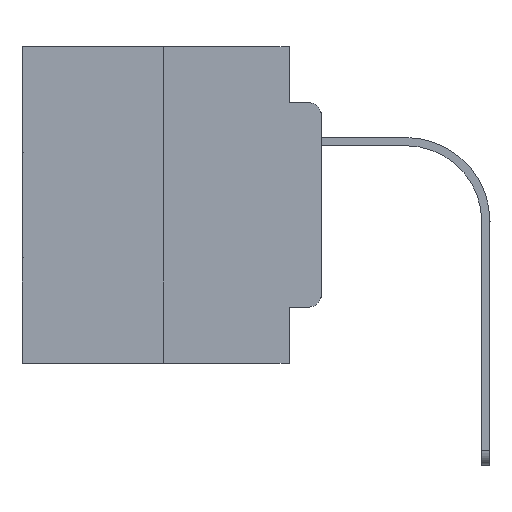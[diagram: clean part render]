
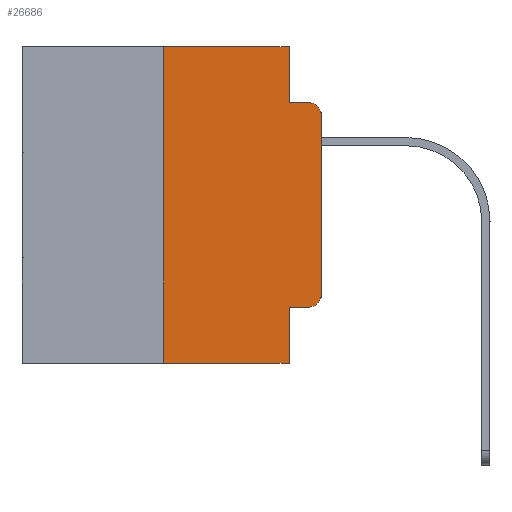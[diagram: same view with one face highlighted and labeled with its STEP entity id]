
A CAD part, left-side view. The second image highlights one B-rep face of the part: STEP entity #26686.
In plain terms, the highlighted planar face has unit normal (-1, 0, 0).
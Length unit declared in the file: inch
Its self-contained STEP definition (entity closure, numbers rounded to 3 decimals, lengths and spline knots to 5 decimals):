
#182 = CARTESIAN_POINT ( 'NONE',  ( 0., 0.051, 0. ) ) ;
#190 = VECTOR ( 'NONE', #3871, 39.37008 ) ;
#312 = CARTESIAN_POINT ( 'NONE',  ( 0., 0.051, -0.4115 ) ) ;
#508 = AXIS2_PLACEMENT_3D ( 'NONE', #15153, #15564, #15695 ) ;
#835 = VERTEX_POINT ( 'NONE', #21291 ) ;
#1941 = VECTOR ( 'NONE', #7481, 39.37008 ) ;
#2773 = VERTEX_POINT ( 'NONE', #18597 ) ;
#3628 = VECTOR ( 'NONE', #14069, 39.37008 ) ;
#3871 = DIRECTION ( 'NONE',  ( 0., 0., 1. ) ) ;
#4007 = EDGE_CURVE ( 'NONE', #23186, #835, #15701, .T. ) ;
#4021 = VECTOR ( 'NONE', #14502, 39.37008 ) ;
#5394 = CARTESIAN_POINT ( 'NONE',  ( 0., 0., -0.3915 ) ) ;
#5417 = AXIS2_PLACEMENT_3D ( 'NONE', #11686, #20808, #22899 ) ;
#5477 = CARTESIAN_POINT ( 'NONE',  ( 0., 0., -0.1085 ) ) ;
#5652 = ORIENTED_EDGE ( 'NONE', *, *, #21293, .T. ) ;
#6458 = ORIENTED_EDGE ( 'NONE', *, *, #24630, .T. ) ;
#6993 = VECTOR ( 'NONE', #22133, 39.37008 ) ;
#7074 = VECTOR ( 'NONE', #24014, 39.37008 ) ;
#7252 = ORIENTED_EDGE ( 'NONE', *, *, #4007, .F. ) ;
#7481 = DIRECTION ( 'NONE',  ( 0., -1., 0. ) ) ;
#7486 = LINE ( 'NONE', #22462, #12081 ) ;
#7670 = CIRCLE ( 'NONE', #15752, 0.02 ) ;
#8280 = VERTEX_POINT ( 'NONE', #21505 ) ;
#8328 = CARTESIAN_POINT ( 'NONE',  ( 0., 0.051, -0.5 ) ) ;
#8457 = ORIENTED_EDGE ( 'NONE', *, *, #16543, .F. ) ;
#8511 = CARTESIAN_POINT ( 'NONE',  ( 0., 0.25, -0.5 ) ) ;
#8588 = LINE ( 'NONE', #12243, #4021 ) ;
#8877 = VERTEX_POINT ( 'NONE', #14450 ) ;
#8885 = LINE ( 'NONE', #182, #7074 ) ;
#9328 = EDGE_CURVE ( 'NONE', #17166, #2773, #25185, .T. ) ;
#9701 = VERTEX_POINT ( 'NONE', #8328 ) ;
#9993 = LINE ( 'NONE', #11668, #1941 ) ;
#11668 = CARTESIAN_POINT ( 'NONE',  ( 0., 0.473, -0.5 ) ) ;
#11686 = CARTESIAN_POINT ( 'NONE',  ( 0., 0.02, -0.3915 ) ) ;
#12081 = VECTOR ( 'NONE', #27126, 39.37008 ) ;
#12243 = CARTESIAN_POINT ( 'NONE',  ( 0., 0.051, 0. ) ) ;
#12506 = ORIENTED_EDGE ( 'NONE', *, *, #19442, .F. ) ;
#12947 = EDGE_CURVE ( 'NONE', #8280, #8877, #22177, .T. ) ;
#13263 = VERTEX_POINT ( 'NONE', #24964 ) ;
#13303 = PLANE ( 'NONE',  #508 ) ;
#14069 = DIRECTION ( 'NONE',  ( 0., 0., 1. ) ) ;
#14192 = ORIENTED_EDGE ( 'NONE', *, *, #19597, .F. ) ;
#14450 = CARTESIAN_POINT ( 'NONE',  ( 0., 0.02, -0.4115 ) ) ;
#14464 = DIRECTION ( 'NONE',  ( 0., 0., -1. ) ) ;
#14502 = DIRECTION ( 'NONE',  ( 0., 0., -1. ) ) ;
#14575 = ORIENTED_EDGE ( 'NONE', *, *, #21854, .T. ) ;
#15153 = CARTESIAN_POINT ( 'NONE',  ( 0., 0.473, 0. ) ) ;
#15564 = DIRECTION ( 'NONE',  ( 1., 0., 0. ) ) ;
#15695 = DIRECTION ( 'NONE',  ( 0., 0., -1. ) ) ;
#15701 = LINE ( 'NONE', #16000, #6993 ) ;
#15752 = AXIS2_PLACEMENT_3D ( 'NONE', #27226, #20905, #14464 ) ;
#16000 = CARTESIAN_POINT ( 'NONE',  ( 0., 0.051, -0.0885 ) ) ;
#16286 = VERTEX_POINT ( 'NONE', #5394 ) ;
#16543 = EDGE_CURVE ( 'NONE', #8280, #9701, #8885, .T. ) ;
#16960 = ORIENTED_EDGE ( 'NONE', *, *, #20641, .T. ) ;
#17166 = VERTEX_POINT ( 'NONE', #8511 ) ;
#18295 = LINE ( 'NONE', #22620, #3628 ) ;
#18597 = CARTESIAN_POINT ( 'NONE',  ( 0., 0.25, 0. ) ) ;
#19406 = CARTESIAN_POINT ( 'NONE',  ( 0., 0.051, -0.0885 ) ) ;
#19442 = EDGE_CURVE ( 'NONE', #2773, #13263, #7486, .T. ) ;
#19597 = EDGE_CURVE ( 'NONE', #13263, #23186, #8588, .T. ) ;
#19880 = VECTOR ( 'NONE', #19940, 39.37008 ) ;
#19940 = DIRECTION ( 'NONE',  ( 0., -1., 0. ) ) ;
#20641 = EDGE_CURVE ( 'NONE', #16286, #26404, #18295, .T. ) ;
#20682 = ORIENTED_EDGE ( 'NONE', *, *, #9328, .F. ) ;
#20808 = DIRECTION ( 'NONE',  ( -1., 0., 0. ) ) ;
#20905 = DIRECTION ( 'NONE',  ( -1., 0., 0. ) ) ;
#21123 = CIRCLE ( 'NONE', #5417, 0.02 ) ;
#21291 = CARTESIAN_POINT ( 'NONE',  ( 0., 0.02, -0.0885 ) ) ;
#21293 = EDGE_CURVE ( 'NONE', #26404, #835, #7670, .T. ) ;
#21505 = CARTESIAN_POINT ( 'NONE',  ( 0., 0.051, -0.4115 ) ) ;
#21854 = EDGE_CURVE ( 'NONE', #8877, #16286, #21123, .T. ) ;
#22133 = DIRECTION ( 'NONE',  ( 0., -1., 0. ) ) ;
#22177 = LINE ( 'NONE', #312, #19880 ) ;
#22305 = EDGE_LOOP ( 'NONE', ( #16960, #5652, #7252, #14192, #12506, #20682, #6458, #8457, #25158, #14575 ) ) ;
#22462 = CARTESIAN_POINT ( 'NONE',  ( 0., 0.473, 0. ) ) ;
#22620 = CARTESIAN_POINT ( 'NONE',  ( 0., 0., 0. ) ) ;
#22899 = DIRECTION ( 'NONE',  ( 0., 0., -1. ) ) ;
#23186 = VERTEX_POINT ( 'NONE', #19406 ) ;
#24014 = DIRECTION ( 'NONE',  ( 0., 0., -1. ) ) ;
#24630 = EDGE_CURVE ( 'NONE', #17166, #9701, #9993, .T. ) ;
#24964 = CARTESIAN_POINT ( 'NONE',  ( 0., 0.051, 0. ) ) ;
#25158 = ORIENTED_EDGE ( 'NONE', *, *, #12947, .T. ) ;
#25185 = LINE ( 'NONE', #25584, #190 ) ;
#25584 = CARTESIAN_POINT ( 'NONE',  ( 0., 0.25, 0. ) ) ;
#26211 = FACE_OUTER_BOUND ( 'NONE', #22305, .T. ) ;
#26404 = VERTEX_POINT ( 'NONE', #5477 ) ;
#26686 = ADVANCED_FACE ( 'NONE', ( #26211 ), #13303, .F. ) ;
#27126 = DIRECTION ( 'NONE',  ( 0., -1., 0. ) ) ;
#27226 = CARTESIAN_POINT ( 'NONE',  ( 0., 0.02, -0.1085 ) ) ;
